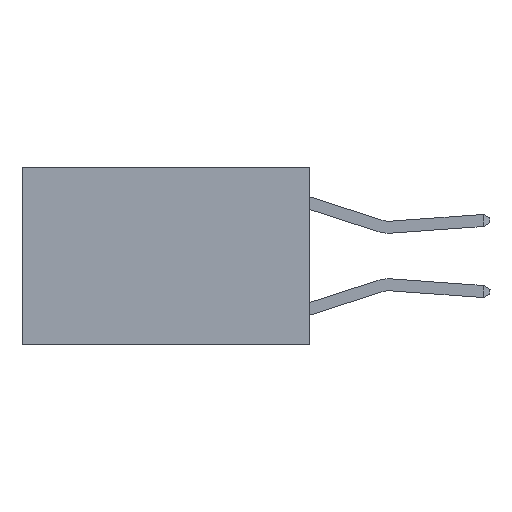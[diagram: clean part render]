
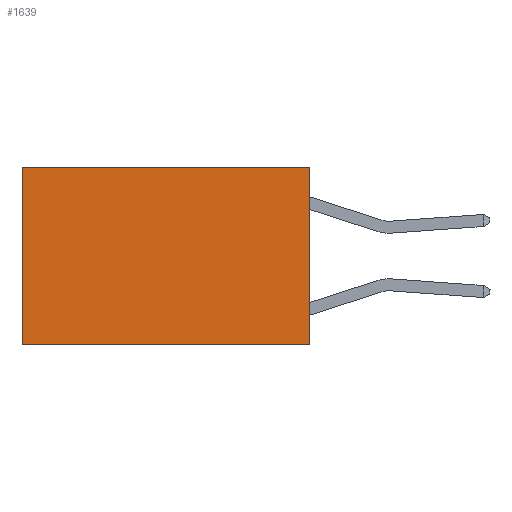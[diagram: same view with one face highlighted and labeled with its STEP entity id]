
A CAD part, left-side view. The second image highlights one B-rep face of the part: STEP entity #1639.
In plain terms, the highlighted planar face has unit normal (-1, 0, 0).
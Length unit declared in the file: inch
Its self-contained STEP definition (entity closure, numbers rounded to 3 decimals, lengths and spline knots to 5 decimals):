
#548 = VERTEX_POINT ( 'NONE', #26077 ) ;
#1639 = ADVANCED_FACE ( 'NONE', ( #6460 ), #27137, .F. ) ;
#1909 = DIRECTION ( 'NONE',  ( 0., 1., 0. ) ) ;
#2093 = LINE ( 'NONE', #6181, #7204 ) ;
#2555 = CARTESIAN_POINT ( 'NONE',  ( 0.2625, 0.6, 0. ) ) ;
#3710 = DIRECTION ( 'NONE',  ( 0., 0., -1. ) ) ;
#4181 = CARTESIAN_POINT ( 'NONE',  ( 0.2625, 0.6, 0. ) ) ;
#5395 = ORIENTED_EDGE ( 'NONE', *, *, #14146, .T. ) ;
#5720 = CARTESIAN_POINT ( 'NONE',  ( 0.2625, 0., 0. ) ) ;
#5977 = VERTEX_POINT ( 'NONE', #4181 ) ;
#6131 = EDGE_CURVE ( 'NONE', #5977, #13661, #13662, .T. ) ;
#6181 = CARTESIAN_POINT ( 'NONE',  ( 0.2625, 0., -0.37 ) ) ;
#6460 = FACE_OUTER_BOUND ( 'NONE', #24407, .T. ) ;
#6465 = LINE ( 'NONE', #8632, #22856 ) ;
#7050 = ORIENTED_EDGE ( 'NONE', *, *, #24871, .F. ) ;
#7110 = CARTESIAN_POINT ( 'NONE',  ( 0.2625, 0., 0. ) ) ;
#7204 = VECTOR ( 'NONE', #1909, 39.37008 ) ;
#7597 = VERTEX_POINT ( 'NONE', #7110 ) ;
#8632 = CARTESIAN_POINT ( 'NONE',  ( 0.2625, 0., 0. ) ) ;
#9456 = ORIENTED_EDGE ( 'NONE', *, *, #6131, .T. ) ;
#10665 = AXIS2_PLACEMENT_3D ( 'NONE', #14536, #16651, #3710 ) ;
#12316 = VECTOR ( 'NONE', #20617, 39.37008 ) ;
#13661 = VERTEX_POINT ( 'NONE', #23447 ) ;
#13662 = LINE ( 'NONE', #2555, #18628 ) ;
#14146 = EDGE_CURVE ( 'NONE', #7597, #5977, #18638, .T. ) ;
#14536 = CARTESIAN_POINT ( 'NONE',  ( 0.2625, 0., 0. ) ) ;
#15070 = EDGE_CURVE ( 'NONE', #7597, #548, #6465, .T. ) ;
#16651 = DIRECTION ( 'NONE',  ( 1., 0., 0. ) ) ;
#17237 = ORIENTED_EDGE ( 'NONE', *, *, #15070, .F. ) ;
#18628 = VECTOR ( 'NONE', #21867, 39.37008 ) ;
#18638 = LINE ( 'NONE', #5720, #12316 ) ;
#19365 = DIRECTION ( 'NONE',  ( 0., 0., -1. ) ) ;
#20617 = DIRECTION ( 'NONE',  ( 0., 1., 0. ) ) ;
#21867 = DIRECTION ( 'NONE',  ( 0., 0., -1. ) ) ;
#22856 = VECTOR ( 'NONE', #19365, 39.37008 ) ;
#23447 = CARTESIAN_POINT ( 'NONE',  ( 0.2625, 0.6, -0.37 ) ) ;
#24407 = EDGE_LOOP ( 'NONE', ( #9456, #7050, #17237, #5395 ) ) ;
#24871 = EDGE_CURVE ( 'NONE', #548, #13661, #2093, .T. ) ;
#26077 = CARTESIAN_POINT ( 'NONE',  ( 0.2625, 0., -0.37 ) ) ;
#27137 = PLANE ( 'NONE',  #10665 ) ;
